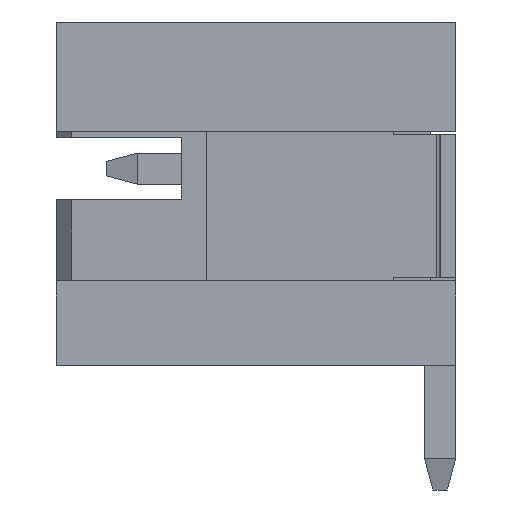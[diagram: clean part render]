
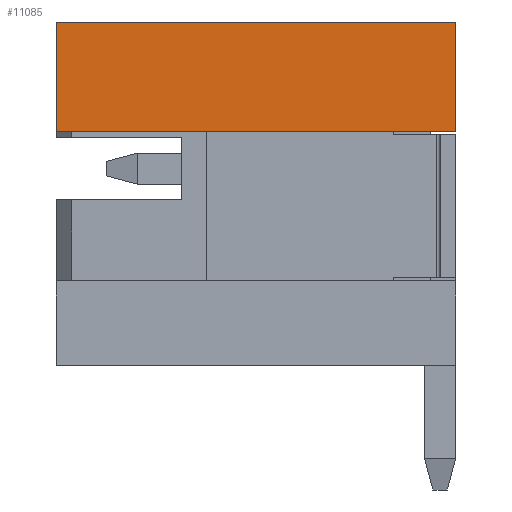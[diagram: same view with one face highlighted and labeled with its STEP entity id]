
A CAD part, left-side view. The second image highlights one B-rep face of the part: STEP entity #11085.
In plain terms, the highlighted planar face has unit normal (-1, 0, 0).
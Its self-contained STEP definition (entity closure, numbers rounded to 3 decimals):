
#255 = VERTEX_POINT ( 'NONE', #3824 ) ;
#1168 = VECTOR ( 'NONE', #2653, 1000. ) ;
#1664 = LINE ( 'NONE', #5844, #3200 ) ;
#1917 = VERTEX_POINT ( 'NONE', #2939 ) ;
#2023 = VERTEX_POINT ( 'NONE', #11212 ) ;
#2303 = AXIS2_PLACEMENT_3D ( 'NONE', #7911, #11320, #3362 ) ;
#2653 = DIRECTION ( 'NONE',  ( 0., 0., -1. ) ) ;
#2939 = CARTESIAN_POINT ( 'NONE',  ( -3., 6.4, 0.6 ) ) ;
#3122 = VECTOR ( 'NONE', #3974, 1000. ) ;
#3200 = VECTOR ( 'NONE', #9467, 1000. ) ;
#3362 = DIRECTION ( 'NONE',  ( 0., 0., -1. ) ) ;
#3525 = ORIENTED_EDGE ( 'NONE', *, *, #4107, .F. ) ;
#3824 = CARTESIAN_POINT ( 'NONE',  ( -3., 0., 0.6 ) ) ;
#3974 = DIRECTION ( 'NONE',  ( 0., -1., 0. ) ) ;
#4063 = ORIENTED_EDGE ( 'NONE', *, *, #7153, .F. ) ;
#4107 = EDGE_CURVE ( 'NONE', #5843, #2023, #4535, .T. ) ;
#4117 = EDGE_LOOP ( 'NONE', ( #7616, #10008, #4063, #3525 ) ) ;
#4143 = CARTESIAN_POINT ( 'NONE',  ( -3., 0., 0.6 ) ) ;
#4196 = PLANE ( 'NONE',  #2303 ) ;
#4535 = LINE ( 'NONE', #6598, #3122 ) ;
#4692 = LINE ( 'NONE', #9475, #1168 ) ;
#4706 = EDGE_CURVE ( 'NONE', #1917, #5843, #1664, .T. ) ;
#5423 = CARTESIAN_POINT ( 'NONE',  ( -3., 6.4, 2.35 ) ) ;
#5843 = VERTEX_POINT ( 'NONE', #5423 ) ;
#5844 = CARTESIAN_POINT ( 'NONE',  ( -3., 6.4, 2.35 ) ) ;
#5956 = EDGE_CURVE ( 'NONE', #255, #1917, #9911, .T. ) ;
#6598 = CARTESIAN_POINT ( 'NONE',  ( -3., 6.4, 2.35 ) ) ;
#7153 = EDGE_CURVE ( 'NONE', #2023, #255, #4692, .T. ) ;
#7499 = VECTOR ( 'NONE', #11185, 1000. ) ;
#7616 = ORIENTED_EDGE ( 'NONE', *, *, #4706, .F. ) ;
#7911 = CARTESIAN_POINT ( 'NONE',  ( -3., 0., 0. ) ) ;
#9467 = DIRECTION ( 'NONE',  ( 0., 0., 1. ) ) ;
#9475 = CARTESIAN_POINT ( 'NONE',  ( -3., 0., 2.35 ) ) ;
#9911 = LINE ( 'NONE', #4143, #7499 ) ;
#10008 = ORIENTED_EDGE ( 'NONE', *, *, #5956, .F. ) ;
#10326 = FACE_OUTER_BOUND ( 'NONE', #4117, .T. ) ;
#11085 = ADVANCED_FACE ( 'NONE', ( #10326 ), #4196, .F. ) ;
#11185 = DIRECTION ( 'NONE',  ( 0., 1., 0. ) ) ;
#11212 = CARTESIAN_POINT ( 'NONE',  ( -3., 0., 2.35 ) ) ;
#11320 = DIRECTION ( 'NONE',  ( 1., 0., 0. ) ) ;
